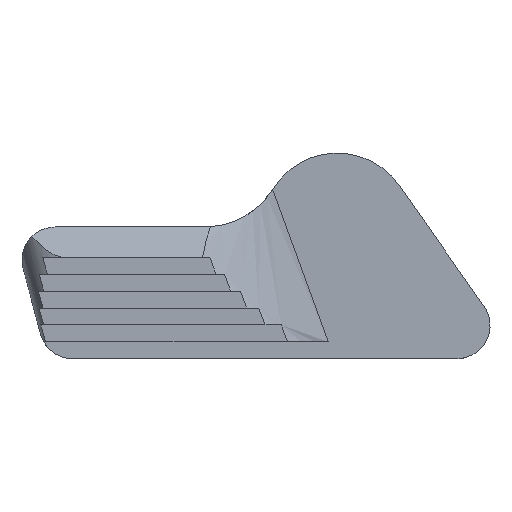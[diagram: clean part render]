
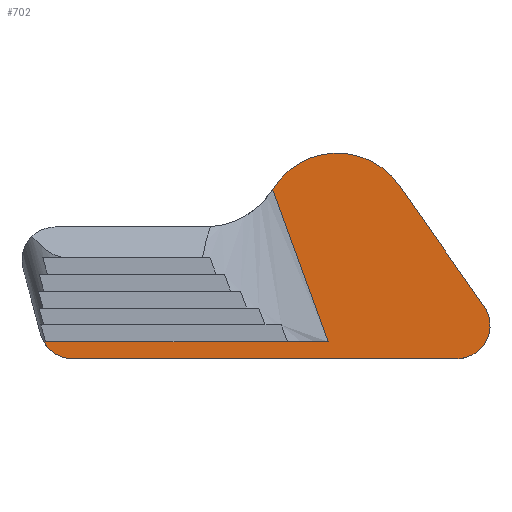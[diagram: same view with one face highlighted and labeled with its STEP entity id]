
A CAD part, top view. The second image highlights one B-rep face of the part: STEP entity #702.
In plain terms, the highlighted planar face has unit normal (0, 0, 1).
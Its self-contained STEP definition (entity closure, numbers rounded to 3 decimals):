
#4 = AXIS2_PLACEMENT_3D ( 'NONE', #1144, #1141, #1138 ) ;
#83 = EDGE_CURVE ( 'NONE', #491, #507, #928, .T. ) ;
#105 = EDGE_CURVE ( 'NONE', #1389, #491, #1422, .T. ) ;
#131 = CIRCLE ( 'NONE', #955, 4.534 ) ;
#157 = CIRCLE ( 'NONE', #988, 1.984 ) ;
#187 = EDGE_CURVE ( 'NONE', #569, #507, #1196, .T. ) ;
#329 = CARTESIAN_POINT ( 'NONE',  ( -15.79, -7.734, 2.184 ) ) ;
#350 = CARTESIAN_POINT ( 'NONE',  ( 8.764, -4.612, 2.184 ) ) ;
#385 = EDGE_CURVE ( 'NONE', #1363, #925, #1172, .T. ) ;
#399 = EDGE_CURVE ( 'NONE', #705, #1363, #157, .T. ) ;
#414 = EDGE_CURVE ( 'NONE', #1389, #705, #1092, .T. ) ;
#416 = EDGE_LOOP ( 'NONE', ( #841, #614, #635, #657, #679, #1170, #1071 ) ) ;
#424 = EDGE_CURVE ( 'NONE', #925, #569, #131, .T. ) ;
#459 = CARTESIAN_POINT ( 'NONE',  ( 3.714, 2.601, 2.184 ) ) ;
#491 = VERTEX_POINT ( 'NONE', #536 ) ;
#500 = VECTOR ( 'NONE', #629, 1000. ) ;
#507 = VERTEX_POINT ( 'NONE', #534 ) ;
#508 = DIRECTION ( 'NONE',  ( 1., 0., 0. ) ) ;
#510 = PLANE ( 'NONE',  #858 ) ;
#512 = CARTESIAN_POINT ( 'NONE',  ( 7.139, -7.734, 2.184 ) ) ;
#513 = CARTESIAN_POINT ( 'NONE',  ( -4.832, -3.347, 2.184 ) ) ;
#514 = DIRECTION ( 'NONE',  ( 0., 0., 1. ) ) ;
#534 = CARTESIAN_POINT ( 'NONE',  ( -0.54, -6.727, 2.184 ) ) ;
#536 = CARTESIAN_POINT ( 'NONE',  ( -17.517, -6.727, 2.184 ) ) ;
#552 = CARTESIAN_POINT ( 'NONE',  ( -3.856, 2.385, 2.184 ) ) ;
#559 = DIRECTION ( 'NONE',  ( 0.819, 0.574, 0. ) ) ;
#561 = DIRECTION ( 'NONE',  ( 0., 0., 1. ) ) ;
#563 = CARTESIAN_POINT ( 'NONE',  ( 0., 0., 2.184 ) ) ;
#569 = VERTEX_POINT ( 'NONE', #552 ) ;
#575 = DIRECTION ( 'NONE',  ( 1., 0., 0. ) ) ;
#590 = VECTOR ( 'NONE', #1176, 1000. ) ;
#599 = DIRECTION ( 'NONE',  ( 0., -1., 0. ) ) ;
#600 = DIRECTION ( 'NONE',  ( 0., 0., 1. ) ) ;
#601 = CARTESIAN_POINT ( 'NONE',  ( 7.139, -5.75, 2.184 ) ) ;
#614 = ORIENTED_EDGE ( 'NONE', *, *, #385, .T. ) ;
#619 = CARTESIAN_POINT ( 'NONE',  ( -15.79, -7.734, 2.184 ) ) ;
#629 = DIRECTION ( 'NONE',  ( -0.574, 0.819, 0. ) ) ;
#631 = CARTESIAN_POINT ( 'NONE',  ( 8.764, -4.612, 2.184 ) ) ;
#635 = ORIENTED_EDGE ( 'NONE', *, *, #424, .T. ) ;
#657 = ORIENTED_EDGE ( 'NONE', *, *, #187, .T. ) ;
#679 = ORIENTED_EDGE ( 'NONE', *, *, #83, .F. ) ;
#702 = ADVANCED_FACE ( 'NONE', ( #768 ), #510, .T. ) ;
#705 = VERTEX_POINT ( 'NONE', #512 ) ;
#768 = FACE_OUTER_BOUND ( 'NONE', #416, .T. ) ;
#841 = ORIENTED_EDGE ( 'NONE', *, *, #399, .T. ) ;
#858 = AXIS2_PLACEMENT_3D ( 'NONE', #513, #514, #508 ) ;
#925 = VERTEX_POINT ( 'NONE', #459 ) ;
#928 = LINE ( 'NONE', #1198, #590 ) ;
#955 = AXIS2_PLACEMENT_3D ( 'NONE', #563, #561, #559 ) ;
#988 = AXIS2_PLACEMENT_3D ( 'NONE', #601, #600, #599 ) ;
#1019 = DIRECTION ( 'NONE',  ( 0.342, -0.94, 0. ) ) ;
#1020 = CARTESIAN_POINT ( 'NONE',  ( -1.151, -5.049, 2.184 ) ) ;
#1055 = VECTOR ( 'NONE', #575, 1000. ) ;
#1071 = ORIENTED_EDGE ( 'NONE', *, *, #414, .T. ) ;
#1092 = LINE ( 'NONE', #619, #1055 ) ;
#1138 = DIRECTION ( 'NONE',  ( -0.966, -0.259, 0. ) ) ;
#1141 = DIRECTION ( 'NONE',  ( 0., 0., -1. ) ) ;
#1144 = CARTESIAN_POINT ( 'NONE',  ( -15.79, -5.75, 2.184 ) ) ;
#1165 = VECTOR ( 'NONE', #1019, 1000. ) ;
#1170 = ORIENTED_EDGE ( 'NONE', *, *, #105, .F. ) ;
#1172 = LINE ( 'NONE', #631, #500 ) ;
#1176 = DIRECTION ( 'NONE',  ( 1., 0., 0. ) ) ;
#1196 = LINE ( 'NONE', #1020, #1165 ) ;
#1198 = CARTESIAN_POINT ( 'NONE',  ( -18.817, -6.727, 2.184 ) ) ;
#1363 = VERTEX_POINT ( 'NONE', #350 ) ;
#1389 = VERTEX_POINT ( 'NONE', #329 ) ;
#1422 = CIRCLE ( 'NONE', #4, 1.984 ) ;
